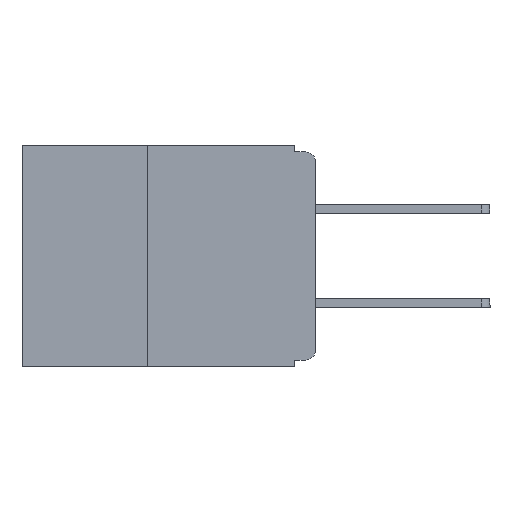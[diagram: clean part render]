
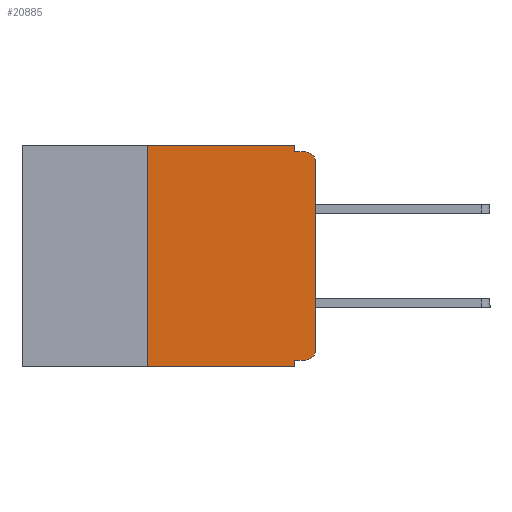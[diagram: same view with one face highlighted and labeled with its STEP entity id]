
A CAD part, left-side view. The second image highlights one B-rep face of the part: STEP entity #20885.
In plain terms, the highlighted planar face has unit normal (-1, 0, 0).
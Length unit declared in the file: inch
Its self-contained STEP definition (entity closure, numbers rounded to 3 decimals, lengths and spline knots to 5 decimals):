
#571 = VECTOR ( 'NONE', #16717, 39.37008 ) ;
#775 = VERTEX_POINT ( 'NONE', #6773 ) ;
#1485 = EDGE_CURVE ( 'NONE', #775, #27419, #24502, .T. ) ;
#1672 = ORIENTED_EDGE ( 'NONE', *, *, #25075, .T. ) ;
#1874 = VECTOR ( 'NONE', #28106, 39.37008 ) ;
#1999 = ORIENTED_EDGE ( 'NONE', *, *, #22119, .F. ) ;
#2627 = VECTOR ( 'NONE', #2699, 39.37008 ) ;
#2643 = ORIENTED_EDGE ( 'NONE', *, *, #1485, .F. ) ;
#2699 = DIRECTION ( 'NONE',  ( 0., 0., 1. ) ) ;
#2981 = CIRCLE ( 'NONE', #19220, 0.015 ) ;
#3171 = PLANE ( 'NONE',  #25074 ) ;
#3346 = CIRCLE ( 'NONE', #17629, 0.015 ) ;
#3372 = LINE ( 'NONE', #9708, #2627 ) ;
#3533 = ORIENTED_EDGE ( 'NONE', *, *, #20852, .T. ) ;
#4310 = ORIENTED_EDGE ( 'NONE', *, *, #7229, .T. ) ;
#4313 = CARTESIAN_POINT ( 'NONE',  ( 0., 0.25, -0.33 ) ) ;
#4721 = ORIENTED_EDGE ( 'NONE', *, *, #25292, .T. ) ;
#4991 = CARTESIAN_POINT ( 'NONE',  ( 0., 0.031, 0. ) ) ;
#5320 = EDGE_LOOP ( 'NONE', ( #4310, #4721, #6651, #6778, #7376, #18785, #1672, #1999, #2643, #3533 ) ) ;
#5965 = CARTESIAN_POINT ( 'NONE',  ( 0., 0., -0.305 ) ) ;
#6121 = VECTOR ( 'NONE', #17208, 39.37008 ) ;
#6651 = ORIENTED_EDGE ( 'NONE', *, *, #14145, .F. ) ;
#6656 = DIRECTION ( 'NONE',  ( 0., 0., 1. ) ) ;
#6773 = CARTESIAN_POINT ( 'NONE',  ( 0., 0.015, -0.32 ) ) ;
#6778 = ORIENTED_EDGE ( 'NONE', *, *, #28026, .F. ) ;
#6954 = LINE ( 'NONE', #16357, #19402 ) ;
#7229 = EDGE_CURVE ( 'NONE', #18560, #17731, #3372, .T. ) ;
#7376 = ORIENTED_EDGE ( 'NONE', *, *, #13991, .F. ) ;
#7480 = CARTESIAN_POINT ( 'NONE',  ( 0., 0.031, -0.32 ) ) ;
#7603 = DIRECTION ( 'NONE',  ( 0., -1., 0. ) ) ;
#7629 = LINE ( 'NONE', #23481, #571 ) ;
#7912 = DIRECTION ( 'NONE',  ( 0., 0., -1. ) ) ;
#8056 = VERTEX_POINT ( 'NONE', #12826 ) ;
#9708 = CARTESIAN_POINT ( 'NONE',  ( 0., 0., 0. ) ) ;
#11396 = VERTEX_POINT ( 'NONE', #24014 ) ;
#11687 = DIRECTION ( 'NONE',  ( 0., -1., 0. ) ) ;
#12401 = CARTESIAN_POINT ( 'NONE',  ( 0., 0.015, -0.305 ) ) ;
#12826 = CARTESIAN_POINT ( 'NONE',  ( 0., 0.015, -0.01 ) ) ;
#13459 = LINE ( 'NONE', #15755, #18919 ) ;
#13545 = CARTESIAN_POINT ( 'NONE',  ( 0., 0.015, -0.025 ) ) ;
#13991 = EDGE_CURVE ( 'NONE', #24765, #28022, #6954, .T. ) ;
#14145 = EDGE_CURVE ( 'NONE', #11396, #8056, #26961, .T. ) ;
#14292 = CARTESIAN_POINT ( 'NONE',  ( 0., 0., -0.025 ) ) ;
#14423 = FACE_OUTER_BOUND ( 'NONE', #5320, .T. ) ;
#14615 = CARTESIAN_POINT ( 'NONE',  ( 0., 0., -0.32 ) ) ;
#14826 = DIRECTION ( 'NONE',  ( 0., 0., -1. ) ) ;
#15130 = VERTEX_POINT ( 'NONE', #22906 ) ;
#15755 = CARTESIAN_POINT ( 'NONE',  ( 0., 0.031, -0.33 ) ) ;
#15918 = DIRECTION ( 'NONE',  ( 0., 0., -1. ) ) ;
#16357 = CARTESIAN_POINT ( 'NONE',  ( 0., 0.437, 0. ) ) ;
#16717 = DIRECTION ( 'NONE',  ( 0., 0., -1. ) ) ;
#16785 = CARTESIAN_POINT ( 'NONE',  ( 0., 0.031, -0.33 ) ) ;
#17208 = DIRECTION ( 'NONE',  ( 0., 1., 0. ) ) ;
#17629 = AXIS2_PLACEMENT_3D ( 'NONE', #12401, #28218, #14826 ) ;
#17642 = VECTOR ( 'NONE', #6656, 39.37008 ) ;
#17731 = VERTEX_POINT ( 'NONE', #14292 ) ;
#17951 = LINE ( 'NONE', #4313, #17642 ) ;
#18560 = VERTEX_POINT ( 'NONE', #5965 ) ;
#18785 = ORIENTED_EDGE ( 'NONE', *, *, #26543, .F. ) ;
#18919 = VECTOR ( 'NONE', #24772, 39.37008 ) ;
#19220 = AXIS2_PLACEMENT_3D ( 'NONE', #13545, #29234, #15918 ) ;
#19244 = CARTESIAN_POINT ( 'NONE',  ( 0., 0., -0.01 ) ) ;
#19402 = VECTOR ( 'NONE', #11687, 39.37008 ) ;
#19547 = CARTESIAN_POINT ( 'NONE',  ( 0., 0.437, 0. ) ) ;
#20524 = LINE ( 'NONE', #25910, #1874 ) ;
#20852 = EDGE_CURVE ( 'NONE', #775, #18560, #3346, .T. ) ;
#20885 = ADVANCED_FACE ( 'NONE', ( #14423 ), #3171, .F. ) ;
#21755 = DIRECTION ( 'NONE',  ( 1., 0., 0. ) ) ;
#21806 = VECTOR ( 'NONE', #7603, 39.37008 ) ;
#22119 = EDGE_CURVE ( 'NONE', #27419, #28628, #13459, .T. ) ;
#22906 = CARTESIAN_POINT ( 'NONE',  ( 0., 0.25, -0.33 ) ) ;
#23481 = CARTESIAN_POINT ( 'NONE',  ( 0., 0.031, 0. ) ) ;
#24014 = CARTESIAN_POINT ( 'NONE',  ( 0., 0.031, -0.01 ) ) ;
#24502 = LINE ( 'NONE', #14615, #6121 ) ;
#24765 = VERTEX_POINT ( 'NONE', #24784 ) ;
#24772 = DIRECTION ( 'NONE',  ( 0., 0., -1. ) ) ;
#24784 = CARTESIAN_POINT ( 'NONE',  ( 0., 0.25, 0. ) ) ;
#25074 = AXIS2_PLACEMENT_3D ( 'NONE', #19547, #21755, #7912 ) ;
#25075 = EDGE_CURVE ( 'NONE', #15130, #28628, #20524, .T. ) ;
#25292 = EDGE_CURVE ( 'NONE', #17731, #8056, #2981, .T. ) ;
#25910 = CARTESIAN_POINT ( 'NONE',  ( 0., 0.437, -0.33 ) ) ;
#26543 = EDGE_CURVE ( 'NONE', #15130, #24765, #17951, .T. ) ;
#26961 = LINE ( 'NONE', #19244, #21806 ) ;
#27419 = VERTEX_POINT ( 'NONE', #7480 ) ;
#28022 = VERTEX_POINT ( 'NONE', #4991 ) ;
#28026 = EDGE_CURVE ( 'NONE', #28022, #11396, #7629, .T. ) ;
#28106 = DIRECTION ( 'NONE',  ( 0., -1., 0. ) ) ;
#28218 = DIRECTION ( 'NONE',  ( -1., 0., 0. ) ) ;
#28628 = VERTEX_POINT ( 'NONE', #16785 ) ;
#29234 = DIRECTION ( 'NONE',  ( -1., 0., 0. ) ) ;
